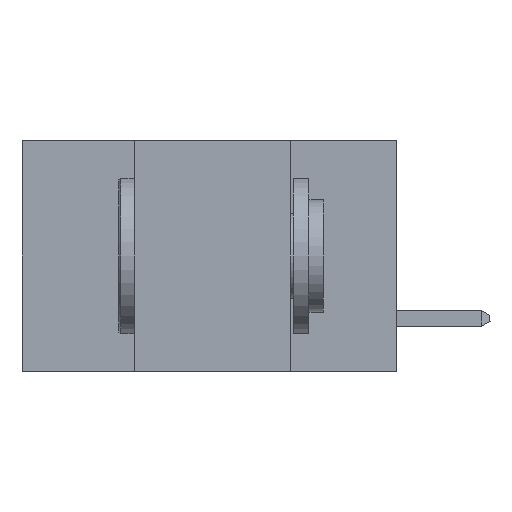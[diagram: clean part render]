
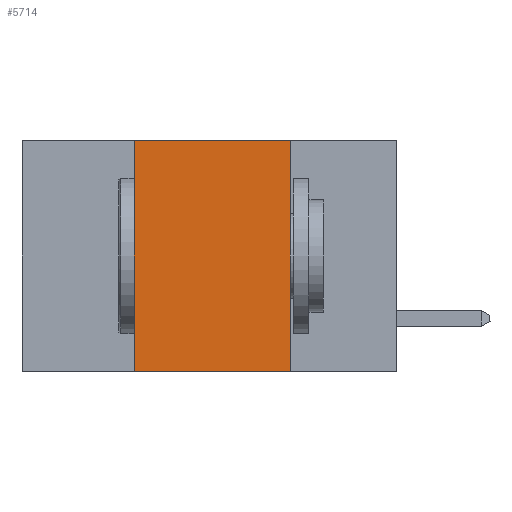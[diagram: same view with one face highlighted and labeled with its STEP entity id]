
A CAD part, left-side view. The second image highlights one B-rep face of the part: STEP entity #5714.
In plain terms, the highlighted planar face has unit normal (-1, 0, 0).
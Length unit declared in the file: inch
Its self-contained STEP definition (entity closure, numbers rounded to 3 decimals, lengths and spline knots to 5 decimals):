
#68 = DIRECTION ( 'NONE',  ( 1., 0., 0. ) ) ;
#181 = EDGE_LOOP ( 'NONE', ( #2471, #13122, #14210, #13101 ) ) ;
#663 = CARTESIAN_POINT ( 'NONE',  ( 0., 0.42, -0.37 ) ) ;
#748 = AXIS2_PLACEMENT_3D ( 'NONE', #12289, #68, #2960 ) ;
#1483 = EDGE_CURVE ( 'NONE', #7384, #4228, #15959, .T. ) ;
#2209 = VECTOR ( 'NONE', #6270, 39.37008 ) ;
#2431 = CARTESIAN_POINT ( 'NONE',  ( 0., 0.17, -0.37 ) ) ;
#2471 = ORIENTED_EDGE ( 'NONE', *, *, #1483, .F. ) ;
#2682 = FACE_OUTER_BOUND ( 'NONE', #181, .T. ) ;
#2960 = DIRECTION ( 'NONE',  ( 0., 0., -1. ) ) ;
#4212 = EDGE_CURVE ( 'NONE', #12242, #4228, #7768, .T. ) ;
#4228 = VERTEX_POINT ( 'NONE', #2431 ) ;
#5494 = CARTESIAN_POINT ( 'NONE',  ( 0., 0.6, -0.37 ) ) ;
#5714 = ADVANCED_FACE ( 'NONE', ( #2682 ), #9033, .F. ) ;
#6270 = DIRECTION ( 'NONE',  ( 0., -1., 0. ) ) ;
#6346 = EDGE_CURVE ( 'NONE', #13468, #7384, #6957, .T. ) ;
#6957 = LINE ( 'NONE', #10914, #2209 ) ;
#7384 = VERTEX_POINT ( 'NONE', #14596 ) ;
#7623 = CARTESIAN_POINT ( 'NONE',  ( 0., 0.42, 0. ) ) ;
#7768 = LINE ( 'NONE', #5494, #11084 ) ;
#8682 = CARTESIAN_POINT ( 'NONE',  ( 0., 0.42, 0. ) ) ;
#8936 = DIRECTION ( 'NONE',  ( 0., 0., 1. ) ) ;
#9033 = PLANE ( 'NONE',  #748 ) ;
#10914 = CARTESIAN_POINT ( 'NONE',  ( 0., 0.6, 0. ) ) ;
#11084 = VECTOR ( 'NONE', #19060, 39.37008 ) ;
#11451 = VECTOR ( 'NONE', #19149, 39.37008 ) ;
#12242 = VERTEX_POINT ( 'NONE', #663 ) ;
#12289 = CARTESIAN_POINT ( 'NONE',  ( 0., 0.6, 0. ) ) ;
#13101 = ORIENTED_EDGE ( 'NONE', *, *, #4212, .T. ) ;
#13122 = ORIENTED_EDGE ( 'NONE', *, *, #6346, .F. ) ;
#13468 = VERTEX_POINT ( 'NONE', #7623 ) ;
#14210 = ORIENTED_EDGE ( 'NONE', *, *, #18235, .F. ) ;
#14596 = CARTESIAN_POINT ( 'NONE',  ( 0., 0.17, 0. ) ) ;
#14845 = LINE ( 'NONE', #8682, #18399 ) ;
#15959 = LINE ( 'NONE', #17557, #11451 ) ;
#17557 = CARTESIAN_POINT ( 'NONE',  ( 0., 0.17, 0. ) ) ;
#18235 = EDGE_CURVE ( 'NONE', #12242, #13468, #14845, .T. ) ;
#18399 = VECTOR ( 'NONE', #8936, 39.37008 ) ;
#19060 = DIRECTION ( 'NONE',  ( 0., -1., 0. ) ) ;
#19149 = DIRECTION ( 'NONE',  ( 0., 0., -1. ) ) ;
